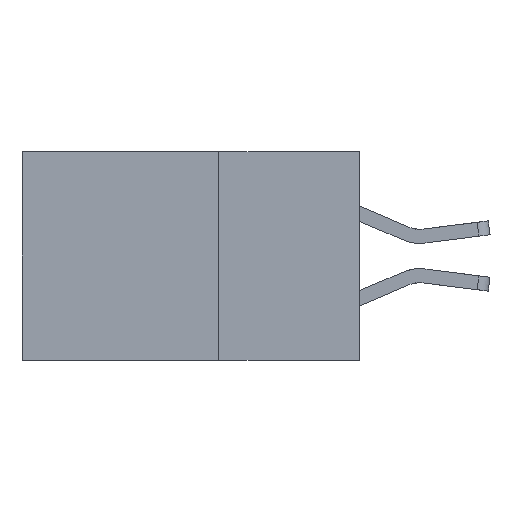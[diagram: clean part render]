
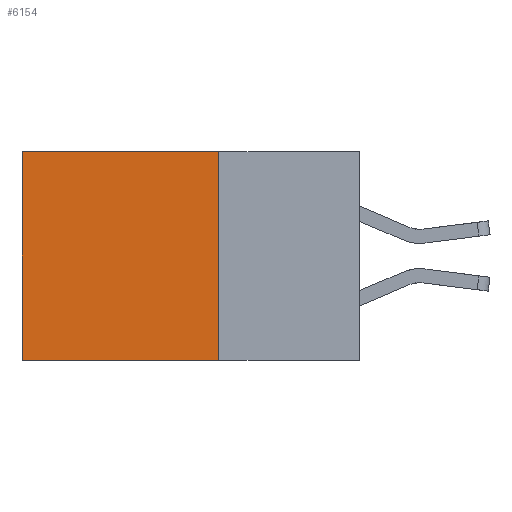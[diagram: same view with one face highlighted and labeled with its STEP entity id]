
A CAD part, left-side view. The second image highlights one B-rep face of the part: STEP entity #6154.
In plain terms, the highlighted planar face has unit normal (-1, 0, 0).
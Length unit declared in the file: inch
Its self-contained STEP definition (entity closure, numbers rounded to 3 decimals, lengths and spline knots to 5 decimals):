
#311 = VERTEX_POINT ( 'NONE', #11215 ) ;
#920 = CARTESIAN_POINT ( 'NONE',  ( 0.2875, 0.25, 0. ) ) ;
#1023 = LINE ( 'NONE', #7578, #4162 ) ;
#1115 = VERTEX_POINT ( 'NONE', #4787 ) ;
#1678 = CARTESIAN_POINT ( 'NONE',  ( 0.2875, 0.6, 0. ) ) ;
#2632 = CARTESIAN_POINT ( 'NONE',  ( 0.2875, 0.25, -0.37 ) ) ;
#2754 = DIRECTION ( 'NONE',  ( 0., 1., 0. ) ) ;
#2845 = DIRECTION ( 'NONE',  ( 0., 0., -1. ) ) ;
#4162 = VECTOR ( 'NONE', #7777, 39.37008 ) ;
#4459 = VECTOR ( 'NONE', #5439, 39.37008 ) ;
#4787 = CARTESIAN_POINT ( 'NONE',  ( 0.2875, 0.6, -0.37 ) ) ;
#5050 = PLANE ( 'NONE',  #9418 ) ;
#5439 = DIRECTION ( 'NONE',  ( 0., 0., -1. ) ) ;
#5454 = EDGE_LOOP ( 'NONE', ( #10752, #5510, #9757, #8770 ) ) ;
#5510 = ORIENTED_EDGE ( 'NONE', *, *, #9475, .F. ) ;
#5592 = VERTEX_POINT ( 'NONE', #11217 ) ;
#5764 = DIRECTION ( 'NONE',  ( 0., 0., -1. ) ) ;
#6063 = EDGE_CURVE ( 'NONE', #5592, #1115, #10161, .T. ) ;
#6154 = ADVANCED_FACE ( 'NONE', ( #8472 ), #5050, .F. ) ;
#6809 = LINE ( 'NONE', #11354, #7744 ) ;
#7119 = VECTOR ( 'NONE', #2754, 39.37008 ) ;
#7478 = DIRECTION ( 'NONE',  ( 1., 0., 0. ) ) ;
#7578 = CARTESIAN_POINT ( 'NONE',  ( 0.2875, 0.25, 0. ) ) ;
#7744 = VECTOR ( 'NONE', #5764, 39.37008 ) ;
#7777 = DIRECTION ( 'NONE',  ( 0., 1., 0. ) ) ;
#8100 = VERTEX_POINT ( 'NONE', #2632 ) ;
#8261 = CARTESIAN_POINT ( 'NONE',  ( 0.2875, 0.25, -0.37 ) ) ;
#8472 = FACE_OUTER_BOUND ( 'NONE', #5454, .T. ) ;
#8770 = ORIENTED_EDGE ( 'NONE', *, *, #9574, .T. ) ;
#9418 = AXIS2_PLACEMENT_3D ( 'NONE', #920, #7478, #2845 ) ;
#9475 = EDGE_CURVE ( 'NONE', #8100, #1115, #11239, .T. ) ;
#9574 = EDGE_CURVE ( 'NONE', #311, #5592, #1023, .T. ) ;
#9757 = ORIENTED_EDGE ( 'NONE', *, *, #9987, .F. ) ;
#9987 = EDGE_CURVE ( 'NONE', #311, #8100, #6809, .T. ) ;
#10161 = LINE ( 'NONE', #1678, #4459 ) ;
#10752 = ORIENTED_EDGE ( 'NONE', *, *, #6063, .T. ) ;
#11215 = CARTESIAN_POINT ( 'NONE',  ( 0.2875, 0.25, 0. ) ) ;
#11217 = CARTESIAN_POINT ( 'NONE',  ( 0.2875, 0.6, 0. ) ) ;
#11239 = LINE ( 'NONE', #8261, #7119 ) ;
#11354 = CARTESIAN_POINT ( 'NONE',  ( 0.2875, 0.25, 0. ) ) ;
